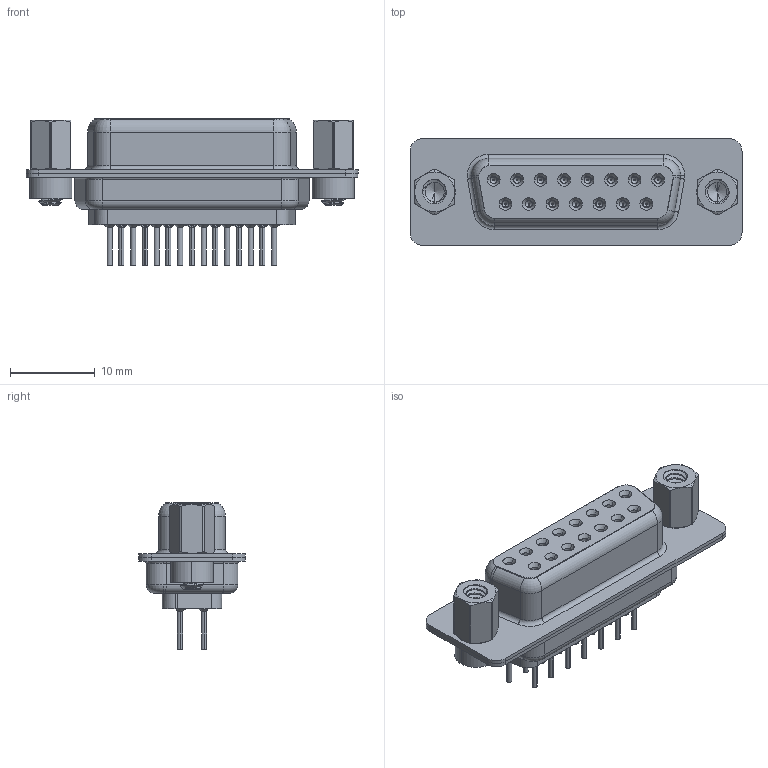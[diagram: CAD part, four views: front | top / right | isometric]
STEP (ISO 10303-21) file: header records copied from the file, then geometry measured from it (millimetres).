
FILE_DESCRIPTION (( 'STEP AP203' ), '1' );
FILE_NAME ('628-015-620-043.STEP', '2020-07-14T02:53:21', ( '' ), ( '' ), 'SwSTEP 2.0', 'SolidWorks 2020', '' );
FILE_SCHEMA (( 'CONFIG_CONTROL_DESIGN' ));
Length unit declared in the file: millimetre
Products named in the file (8): 628 Shell Rear_15 Contacts; 628 Shell Front_15 Contacts; 628 Contact Row 1_20L; 628 4-40 Hex Standoff; 628-015-620-043; 628 Contact Row 2_20L; 628 4-40 Threaded Rivet; 628 Housing_15 LP
Assembly tree (22 placements, depth 2):
  628-015-620-043
    628 Housing_15 LP
    628 Shell Front_15 Contacts
    628 Shell Rear_15 Contacts
    628 Contact Row 1_20L  x8
    628 Contact Row 2_20L  x7
    628 4-40 Threaded Rivet  x2
    628 4-40 Hex Standoff  x2
Bounding box: 39.15 x 12.6 x 17.3 mm (x, y, z)
Volume: 2750.2 mm3; surface area: 6797.8 mm2
Topology: 22 solids, 22 shells, 2306 faces, 5883 edges, 3662 vertices
Faces by surface type: cylinder 702, plane 554, torus 447, bspline 318, cone 285
Entity records: 28701 total; most frequent: CARTESIAN_POINT 10539, DIRECTION 3603, ORIENTED_EDGE 3546, EDGE_CURVE 1773, AXIS2_PLACEMENT_3D 1492, VERTEX_POINT 1117, EDGE_LOOP 826, CIRCLE 790
